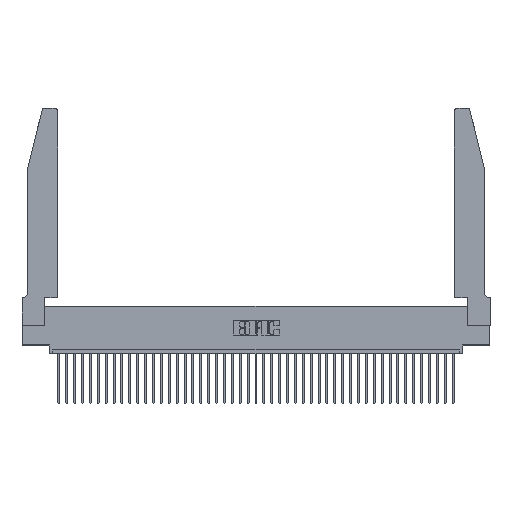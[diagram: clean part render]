
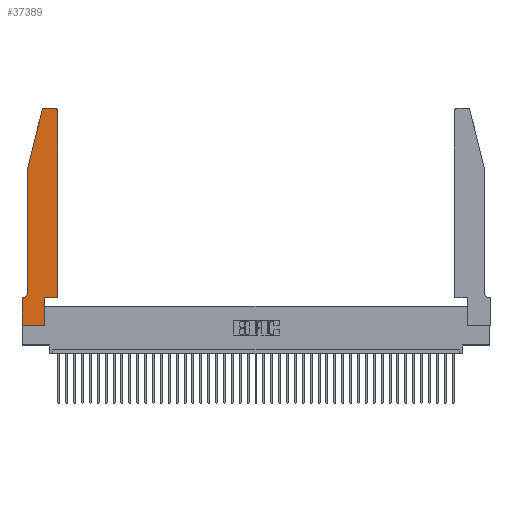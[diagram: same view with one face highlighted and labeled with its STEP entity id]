
A CAD part, top view. The second image highlights one B-rep face of the part: STEP entity #37389.
In plain terms, the highlighted planar face has unit normal (0, 0, 1).
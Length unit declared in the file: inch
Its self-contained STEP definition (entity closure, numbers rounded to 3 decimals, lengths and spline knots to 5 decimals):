
#62 = CARTESIAN_POINT ( 'NONE',  ( 0.4505, 0.35, 0.37 ) ) ;
#230 = DIRECTION ( 'NONE',  ( -0.239, -0.971, 0. ) ) ;
#431 = LINE ( 'NONE', #35445, #15077 ) ;
#495 = EDGE_CURVE ( 'NONE', #20650, #16672, #431, .T. ) ;
#689 = EDGE_CURVE ( 'NONE', #24415, #18325, #14071, .T. ) ;
#836 = VECTOR ( 'NONE', #3305, 39.37008 ) ;
#1012 = DIRECTION ( 'NONE',  ( -1., 0., 0. ) ) ;
#1138 = DIRECTION ( 'NONE',  ( 1., 0., 0. ) ) ;
#2726 = ORIENTED_EDGE ( 'NONE', *, *, #23958, .T. ) ;
#2736 = DIRECTION ( 'NONE',  ( 0., -1., 0. ) ) ;
#3087 = CARTESIAN_POINT ( 'NONE',  ( 0.4505, 0.35, 0.37 ) ) ;
#3128 = CARTESIAN_POINT ( 'NONE',  ( 0.2865, 0., 0.37 ) ) ;
#3193 = CARTESIAN_POINT ( 'NONE',  ( 0.0755, 2., 0.37 ) ) ;
#3305 = DIRECTION ( 'NONE',  ( 1., 0., 0. ) ) ;
#3971 = EDGE_CURVE ( 'NONE', #10857, #36619, #41507, .T. ) ;
#4257 = DIRECTION ( 'NONE',  ( 0., 0., 1. ) ) ;
#5402 = VECTOR ( 'NONE', #230, 39.37008 ) ;
#6225 = LINE ( 'NONE', #28818, #39797 ) ;
#7102 = CIRCLE ( 'NONE', #22628, 0.03 ) ;
#8029 = VECTOR ( 'NONE', #8843, 39.37008 ) ;
#8052 = CARTESIAN_POINT ( 'NONE',  ( 0., 0., 0.37 ) ) ;
#8843 = DIRECTION ( 'NONE',  ( 0., 1., 0. ) ) ;
#10165 = AXIS2_PLACEMENT_3D ( 'NONE', #21684, #41493, #18855 ) ;
#10857 = VERTEX_POINT ( 'NONE', #17763 ) ;
#11247 = VECTOR ( 'NONE', #31865, 39.37008 ) ;
#11452 = CARTESIAN_POINT ( 'NONE',  ( 0., 0.35, 0.37 ) ) ;
#12169 = ORIENTED_EDGE ( 'NONE', *, *, #24867, .T. ) ;
#13439 = EDGE_CURVE ( 'NONE', #25695, #24415, #27472, .T. ) ;
#14071 = LINE ( 'NONE', #21560, #8029 ) ;
#14254 = VERTEX_POINT ( 'NONE', #20278 ) ;
#14857 = ORIENTED_EDGE ( 'NONE', *, *, #13439, .T. ) ;
#15077 = VECTOR ( 'NONE', #29149, 39.37008 ) ;
#15452 = EDGE_CURVE ( 'NONE', #14254, #30700, #32772, .T. ) ;
#15648 = ORIENTED_EDGE ( 'NONE', *, *, #495, .T. ) ;
#16672 = VERTEX_POINT ( 'NONE', #18277 ) ;
#16879 = ORIENTED_EDGE ( 'NONE', *, *, #19151, .T. ) ;
#17763 = CARTESIAN_POINT ( 'NONE',  ( 0.25487, 2.72718, 0.37 ) ) ;
#17833 = VECTOR ( 'NONE', #2736, 39.37008 ) ;
#18208 = ORIENTED_EDGE ( 'NONE', *, *, #33522, .T. ) ;
#18277 = CARTESIAN_POINT ( 'NONE',  ( 0.4505, 2.72, 0.37 ) ) ;
#18325 = VERTEX_POINT ( 'NONE', #32680 ) ;
#18653 = CARTESIAN_POINT ( 'NONE',  ( 0.4205, 2.75, 0.37 ) ) ;
#18855 = DIRECTION ( 'NONE',  ( 1., 0., 0. ) ) ;
#19151 = EDGE_CURVE ( 'NONE', #16672, #32577, #30986, .T. ) ;
#19540 = VECTOR ( 'NONE', #26567, 39.37008 ) ;
#19942 = CARTESIAN_POINT ( 'NONE',  ( 0., 0., 0.37 ) ) ;
#20192 = VECTOR ( 'NONE', #36319, 39.37008 ) ;
#20217 = EDGE_CURVE ( 'NONE', #33060, #14254, #34468, .T. ) ;
#20257 = CARTESIAN_POINT ( 'NONE',  ( 0.0055, 0.42, 0.37 ) ) ;
#20278 = CARTESIAN_POINT ( 'NONE',  ( 0.0055, 0.35, 0.37 ) ) ;
#20650 = VERTEX_POINT ( 'NONE', #3087 ) ;
#21275 = CARTESIAN_POINT ( 'NONE',  ( 0.284, 2.75, 0.37 ) ) ;
#21283 = ORIENTED_EDGE ( 'NONE', *, *, #689, .T. ) ;
#21560 = CARTESIAN_POINT ( 'NONE',  ( 0.2865, 0.35, 0.37 ) ) ;
#21684 = CARTESIAN_POINT ( 'NONE',  ( 0., 0.35, 0.37 ) ) ;
#22142 = CARTESIAN_POINT ( 'NONE',  ( 0.0755, 2., 0.37 ) ) ;
#22628 = AXIS2_PLACEMENT_3D ( 'NONE', #23929, #4257, #1138 ) ;
#22841 = FACE_OUTER_BOUND ( 'NONE', #34161, .T. ) ;
#23929 = CARTESIAN_POINT ( 'NONE',  ( 0.284, 2.72, 0.37 ) ) ;
#23958 = EDGE_CURVE ( 'NONE', #36619, #33060, #24954, .T. ) ;
#24415 = VERTEX_POINT ( 'NONE', #3128 ) ;
#24867 = EDGE_CURVE ( 'NONE', #39153, #10857, #7102, .T. ) ;
#24954 = LINE ( 'NONE', #22142, #17833 ) ;
#25695 = VERTEX_POINT ( 'NONE', #27566 ) ;
#26567 = DIRECTION ( 'NONE',  ( -1., 0., 0. ) ) ;
#27472 = LINE ( 'NONE', #8052, #11247 ) ;
#27566 = CARTESIAN_POINT ( 'NONE',  ( 0., 0., 0.37 ) ) ;
#28529 = ORIENTED_EDGE ( 'NONE', *, *, #15452, .T. ) ;
#28818 = CARTESIAN_POINT ( 'NONE',  ( 0.2605, 2.75, 0.37 ) ) ;
#29149 = DIRECTION ( 'NONE',  ( 0., 1., 0. ) ) ;
#29573 = CARTESIAN_POINT ( 'NONE',  ( 0.0755, 0.35, 0.37 ) ) ;
#29764 = LINE ( 'NONE', #62, #836 ) ;
#30596 = CARTESIAN_POINT ( 'NONE',  ( 0.0755, 2., 0.37 ) ) ;
#30700 = VERTEX_POINT ( 'NONE', #11452 ) ;
#30986 = CIRCLE ( 'NONE', #41821, 0.03 ) ;
#31599 = ORIENTED_EDGE ( 'NONE', *, *, #20217, .T. ) ;
#31865 = DIRECTION ( 'NONE',  ( 1., 0., 0. ) ) ;
#32577 = VERTEX_POINT ( 'NONE', #18653 ) ;
#32680 = CARTESIAN_POINT ( 'NONE',  ( 0.2865, 0.35, 0.37 ) ) ;
#32772 = LINE ( 'NONE', #29573, #19540 ) ;
#32870 = DIRECTION ( 'NONE',  ( 1., 0., 0. ) ) ;
#33060 = VERTEX_POINT ( 'NONE', #37280 ) ;
#33298 = DIRECTION ( 'NONE',  ( 0., 0., 1. ) ) ;
#33522 = EDGE_CURVE ( 'NONE', #18325, #20650, #29764, .T. ) ;
#33568 = ORIENTED_EDGE ( 'NONE', *, *, #3971, .T. ) ;
#34161 = EDGE_LOOP ( 'NONE', ( #35585, #12169, #33568, #2726, #31599, #28529, #41140, #14857, #21283, #18208, #15648, #16879 ) ) ;
#34468 = CIRCLE ( 'NONE', #37784, 0.07 ) ;
#35445 = CARTESIAN_POINT ( 'NONE',  ( 0.4505, 0.35, 0.37 ) ) ;
#35585 = ORIENTED_EDGE ( 'NONE', *, *, #36061, .T. ) ;
#36017 = LINE ( 'NONE', #19942, #20192 ) ;
#36061 = EDGE_CURVE ( 'NONE', #32577, #39153, #6225, .T. ) ;
#36319 = DIRECTION ( 'NONE',  ( 0., -1., 0. ) ) ;
#36619 = VERTEX_POINT ( 'NONE', #30596 ) ;
#36775 = DIRECTION ( 'NONE',  ( 0., 0., -1. ) ) ;
#37280 = CARTESIAN_POINT ( 'NONE',  ( 0.0755, 0.42, 0.37 ) ) ;
#37389 = ADVANCED_FACE ( 'NONE', ( #22841 ), #41200, .T. ) ;
#37784 = AXIS2_PLACEMENT_3D ( 'NONE', #20257, #36775, #1012 ) ;
#38100 = DIRECTION ( 'NONE',  ( -1., 0., 0. ) ) ;
#38424 = EDGE_CURVE ( 'NONE', #30700, #25695, #36017, .T. ) ;
#39153 = VERTEX_POINT ( 'NONE', #21275 ) ;
#39272 = CARTESIAN_POINT ( 'NONE',  ( 0.4205, 2.72, 0.37 ) ) ;
#39797 = VECTOR ( 'NONE', #38100, 39.37008 ) ;
#41140 = ORIENTED_EDGE ( 'NONE', *, *, #38424, .T. ) ;
#41200 = PLANE ( 'NONE',  #10165 ) ;
#41493 = DIRECTION ( 'NONE',  ( 0., 0., 1. ) ) ;
#41507 = LINE ( 'NONE', #3193, #5402 ) ;
#41821 = AXIS2_PLACEMENT_3D ( 'NONE', #39272, #33298, #32870 ) ;
